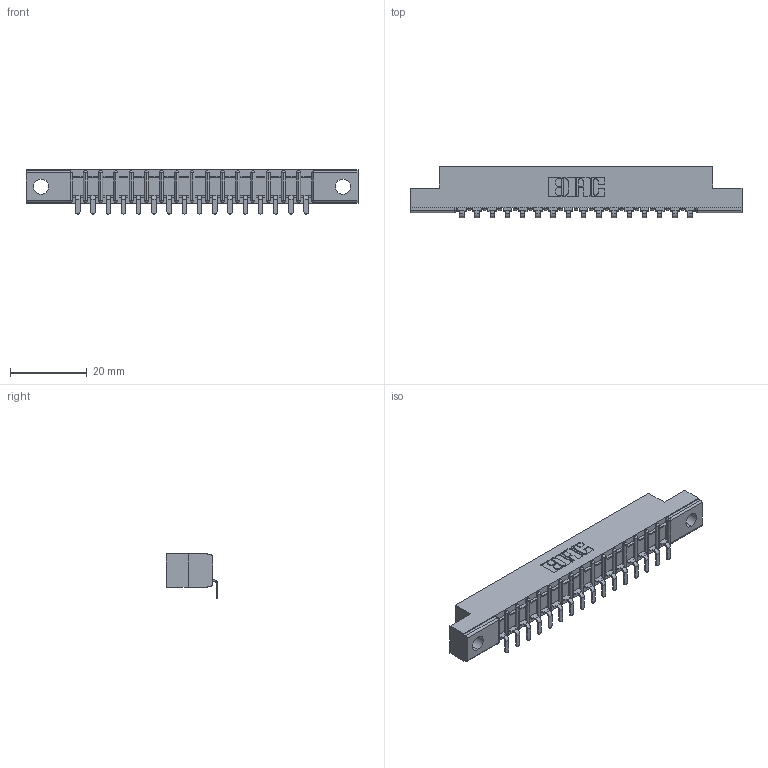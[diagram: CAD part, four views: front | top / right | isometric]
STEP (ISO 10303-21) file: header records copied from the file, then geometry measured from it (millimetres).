
FILE_DESCRIPTION (( 'STEP AP203' ), '1' );
FILE_NAME ('357-016-453-104.STEP', '2020-09-30T20:00:06', ( '' ), ( '' ), 'SwSTEP 2.0', 'SolidWorks 2020', '' );
FILE_SCHEMA (( 'CONFIG_CONTROL_DESIGN' ));
Length unit declared in the file: inch
Products named in the file (3): 357-016-453-104; 307-290-002_553; 307 Part_.156 Dia Mounting Holes
Assembly tree (17 placements, depth 2):
  357-016-453-104
    307 Part_.156 Dia Mounting Holes
    307-290-002_553  x16
Bounding box: 86.41 x 13.32 x 11.51 mm (x, y, z)
Volume: 5595.5 mm3; surface area: 9739.3 mm2
Topology: 17 solids, 17 shells, 1397 faces, 4263 edges, 2794 vertices
Faces by surface type: plane 836, cylinder 527, sphere 34
Entity records: 18194 total; most frequent: CARTESIAN_POINT 3070, ORIENTED_EDGE 3058, DIRECTION 2987, EDGE_CURVE 1529, VECTOR 1165, LINE 1165, VERTEX_POINT 994, AXIS2_PLACEMENT_3D 911
